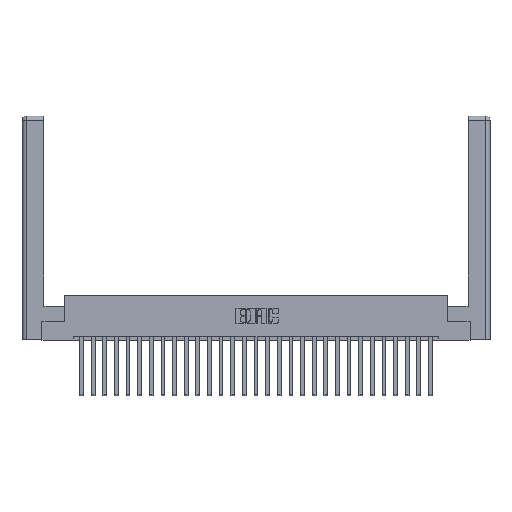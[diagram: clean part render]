
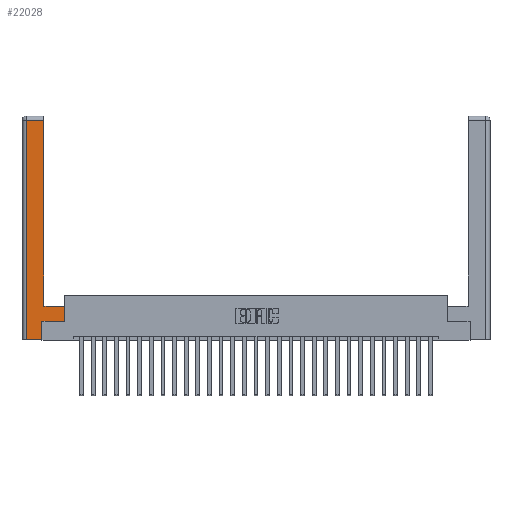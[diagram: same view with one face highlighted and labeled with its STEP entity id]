
A CAD part, top view. The second image highlights one B-rep face of the part: STEP entity #22028.
In plain terms, the highlighted planar face has unit normal (0, 0, 1).
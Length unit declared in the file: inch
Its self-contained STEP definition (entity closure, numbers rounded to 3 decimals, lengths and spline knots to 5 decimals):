
#30 = DIRECTION ( 'NONE',  ( 1., 0., 0. ) ) ;
#211 = ORIENTED_EDGE ( 'NONE', *, *, #22715, .T. ) ;
#902 = VECTOR ( 'NONE', #24754, 39.37008 ) ;
#1061 = CARTESIAN_POINT ( 'NONE',  ( 0., 0., 0. ) ) ;
#1795 = LINE ( 'NONE', #6554, #24066 ) ;
#3211 = DIRECTION ( 'NONE',  ( -1., 0., 0. ) ) ;
#5103 = EDGE_CURVE ( 'NONE', #25210, #14448, #7245, .T. ) ;
#5240 = CARTESIAN_POINT ( 'NONE',  ( 0.295, 3., 0. ) ) ;
#5555 = ORIENTED_EDGE ( 'NONE', *, *, #5103, .T. ) ;
#6097 = DIRECTION ( 'NONE',  ( 0., 1., 0. ) ) ;
#6417 = AXIS2_PLACEMENT_3D ( 'NONE', #1061, #13622, #3211 ) ;
#6554 = CARTESIAN_POINT ( 'NONE',  ( 0.0615, 0., 0. ) ) ;
#6905 = DIRECTION ( 'NONE',  ( 1., 0., 0. ) ) ;
#7245 = LINE ( 'NONE', #17309, #8918 ) ;
#7247 = EDGE_CURVE ( 'NONE', #8767, #22271, #8973, .T. ) ;
#7284 = VERTEX_POINT ( 'NONE', #7772 ) ;
#7772 = CARTESIAN_POINT ( 'NONE',  ( 0.565, 0.45, 0. ) ) ;
#7803 = ORIENTED_EDGE ( 'NONE', *, *, #20592, .T. ) ;
#8058 = DIRECTION ( 'NONE',  ( -1., 0., 0. ) ) ;
#8767 = VERTEX_POINT ( 'NONE', #21740 ) ;
#8918 = VECTOR ( 'NONE', #30, 39.37008 ) ;
#8973 = LINE ( 'NONE', #5240, #902 ) ;
#9074 = VECTOR ( 'NONE', #21801, 39.37008 ) ;
#9269 = VECTOR ( 'NONE', #8058, 39.37008 ) ;
#9718 = VERTEX_POINT ( 'NONE', #25779 ) ;
#10247 = CARTESIAN_POINT ( 'NONE',  ( 0.0615, 0., 0. ) ) ;
#10425 = VERTEX_POINT ( 'NONE', #10247 ) ;
#10641 = EDGE_CURVE ( 'NONE', #10425, #22286, #18437, .T. ) ;
#11098 = CARTESIAN_POINT ( 'NONE',  ( 0.0615, 2.94, 0. ) ) ;
#11899 = CARTESIAN_POINT ( 'NONE',  ( 0.565, 0.245, 0. ) ) ;
#12720 = EDGE_CURVE ( 'NONE', #9718, #10425, #1795, .T. ) ;
#13438 = ORIENTED_EDGE ( 'NONE', *, *, #7247, .T. ) ;
#13471 = LINE ( 'NONE', #13476, #17181 ) ;
#13476 = CARTESIAN_POINT ( 'NONE',  ( 0.265, 0.245, 0. ) ) ;
#13622 = DIRECTION ( 'NONE',  ( 0., 0., -1. ) ) ;
#13907 = PLANE ( 'NONE',  #6417 ) ;
#14075 = FACE_OUTER_BOUND ( 'NONE', #23788, .T. ) ;
#14448 = VERTEX_POINT ( 'NONE', #11899 ) ;
#15649 = DIRECTION ( 'NONE',  ( 0., 1., 0. ) ) ;
#15855 = LINE ( 'NONE', #11098, #9074 ) ;
#16696 = CARTESIAN_POINT ( 'NONE',  ( 0.565, 0.45, 0. ) ) ;
#16719 = CARTESIAN_POINT ( 'NONE',  ( 0.265, 0., 0. ) ) ;
#16900 = CARTESIAN_POINT ( 'NONE',  ( 0.295, 2.94, 0. ) ) ;
#17181 = VECTOR ( 'NONE', #15649, 39.37008 ) ;
#17309 = CARTESIAN_POINT ( 'NONE',  ( 0.565, 0.245, 0. ) ) ;
#17340 = LINE ( 'NONE', #16696, #18323 ) ;
#17644 = EDGE_CURVE ( 'NONE', #14448, #7284, #17340, .T. ) ;
#18323 = VECTOR ( 'NONE', #6097, 39.37008 ) ;
#18437 = LINE ( 'NONE', #22458, #23462 ) ;
#18954 = ORIENTED_EDGE ( 'NONE', *, *, #17644, .T. ) ;
#20217 = EDGE_CURVE ( 'NONE', #22271, #9718, #15855, .T. ) ;
#20592 = EDGE_CURVE ( 'NONE', #22286, #25210, #13471, .T. ) ;
#20744 = LINE ( 'NONE', #23129, #9269 ) ;
#21101 = ORIENTED_EDGE ( 'NONE', *, *, #10641, .T. ) ;
#21740 = CARTESIAN_POINT ( 'NONE',  ( 0.295, 0.45, 0. ) ) ;
#21801 = DIRECTION ( 'NONE',  ( -1., 0., 0. ) ) ;
#22028 = ADVANCED_FACE ( 'NONE', ( #14075 ), #13907, .F. ) ;
#22271 = VERTEX_POINT ( 'NONE', #16900 ) ;
#22286 = VERTEX_POINT ( 'NONE', #16719 ) ;
#22458 = CARTESIAN_POINT ( 'NONE',  ( 0.265, 0., 0. ) ) ;
#22715 = EDGE_CURVE ( 'NONE', #7284, #8767, #20744, .T. ) ;
#23129 = CARTESIAN_POINT ( 'NONE',  ( 0.295, 0.45, 0. ) ) ;
#23417 = DIRECTION ( 'NONE',  ( 0., -1., 0. ) ) ;
#23462 = VECTOR ( 'NONE', #6905, 39.37008 ) ;
#23788 = EDGE_LOOP ( 'NONE', ( #13438, #26076, #26868, #21101, #7803, #5555, #18954, #211 ) ) ;
#24066 = VECTOR ( 'NONE', #23417, 39.37008 ) ;
#24754 = DIRECTION ( 'NONE',  ( 0., 1., 0. ) ) ;
#25210 = VERTEX_POINT ( 'NONE', #26173 ) ;
#25779 = CARTESIAN_POINT ( 'NONE',  ( 0.0615, 2.94, 0. ) ) ;
#26076 = ORIENTED_EDGE ( 'NONE', *, *, #20217, .T. ) ;
#26173 = CARTESIAN_POINT ( 'NONE',  ( 0.265, 0.245, 0. ) ) ;
#26868 = ORIENTED_EDGE ( 'NONE', *, *, #12720, .T. ) ;
